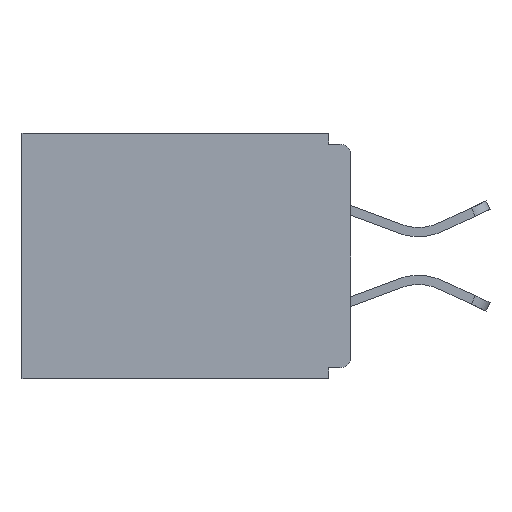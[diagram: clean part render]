
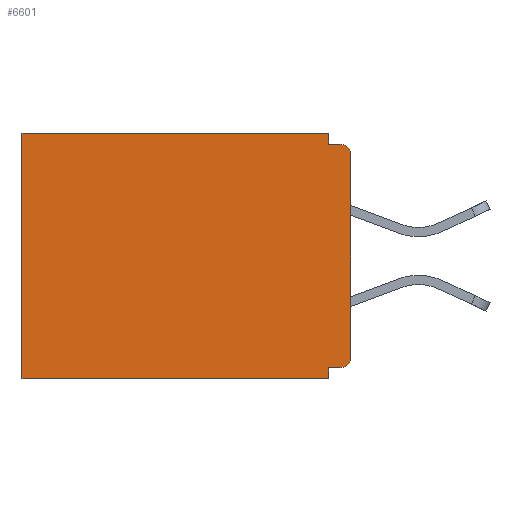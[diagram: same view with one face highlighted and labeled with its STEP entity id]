
A CAD part, left-side view. The second image highlights one B-rep face of the part: STEP entity #6601.
In plain terms, the highlighted planar face has unit normal (-1, 0, 0).
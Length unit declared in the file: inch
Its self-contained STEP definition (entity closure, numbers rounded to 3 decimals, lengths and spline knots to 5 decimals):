
#123 = ORIENTED_EDGE ( 'NONE', *, *, #4149, .T. ) ;
#448 = LINE ( 'NONE', #15597, #10833 ) ;
#1018 = VERTEX_POINT ( 'NONE', #11713 ) ;
#1474 = EDGE_CURVE ( 'NONE', #13057, #2625, #13930, .T. ) ;
#1483 = EDGE_CURVE ( 'NONE', #7050, #9009, #9162, .T. ) ;
#1697 = VECTOR ( 'NONE', #12200, 39.37008 ) ;
#1750 = ORIENTED_EDGE ( 'NONE', *, *, #1483, .F. ) ;
#1841 = CARTESIAN_POINT ( 'NONE',  ( 0.298, 0., 0. ) ) ;
#1875 = VERTEX_POINT ( 'NONE', #3403 ) ;
#2086 = VERTEX_POINT ( 'NONE', #8594 ) ;
#2167 = ORIENTED_EDGE ( 'NONE', *, *, #2631, .F. ) ;
#2180 = CARTESIAN_POINT ( 'NONE',  ( 0.298, 0.46, -0.343 ) ) ;
#2319 = EDGE_CURVE ( 'NONE', #2086, #2996, #7268, .T. ) ;
#2546 = CARTESIAN_POINT ( 'NONE',  ( 0.298, 0., -0.015 ) ) ;
#2625 = VERTEX_POINT ( 'NONE', #5734 ) ;
#2631 = EDGE_CURVE ( 'NONE', #13057, #6788, #15055, .T. ) ;
#2850 = LINE ( 'NONE', #2546, #1697 ) ;
#2859 = EDGE_CURVE ( 'NONE', #1018, #2996, #11800, .T. ) ;
#2996 = VERTEX_POINT ( 'NONE', #11262 ) ;
#3275 = EDGE_CURVE ( 'NONE', #2086, #15191, #10846, .T. ) ;
#3403 = CARTESIAN_POINT ( 'NONE',  ( 0.298, 0.015, -0.015 ) ) ;
#3463 = DIRECTION ( 'NONE',  ( 0., 1., 0. ) ) ;
#3483 = DIRECTION ( 'NONE',  ( 0., 0., -1. ) ) ;
#3580 = CARTESIAN_POINT ( 'NONE',  ( 0.298, 0.015, -0.313 ) ) ;
#4040 = LINE ( 'NONE', #11804, #10444 ) ;
#4149 = EDGE_CURVE ( 'NONE', #1018, #1875, #11959, .T. ) ;
#4512 = DIRECTION ( 'NONE',  ( -1., 0., 0. ) ) ;
#4696 = CARTESIAN_POINT ( 'NONE',  ( 0.298, 0., 0. ) ) ;
#4710 = DIRECTION ( 'NONE',  ( 0., 0., -1. ) ) ;
#5500 = CARTESIAN_POINT ( 'NONE',  ( 0.298, 0.031, -0.015 ) ) ;
#5665 = ORIENTED_EDGE ( 'NONE', *, *, #2319, .T. ) ;
#5734 = CARTESIAN_POINT ( 'NONE',  ( 0.298, 0.46, 0. ) ) ;
#5794 = DIRECTION ( 'NONE',  ( 0., 1., 0. ) ) ;
#5813 = DIRECTION ( 'NONE',  ( -1., 0., 0. ) ) ;
#6601 = ADVANCED_FACE ( 'NONE', ( #8647 ), #6876, .F. ) ;
#6788 = VERTEX_POINT ( 'NONE', #5500 ) ;
#6876 = PLANE ( 'NONE',  #10411 ) ;
#7050 = VERTEX_POINT ( 'NONE', #12848 ) ;
#7137 = EDGE_LOOP ( 'NONE', ( #123, #11182, #2167, #12287, #9486, #1750, #15047, #9133, #5665, #9840 ) ) ;
#7268 = CIRCLE ( 'NONE', #7648, 0.015 ) ;
#7577 = CARTESIAN_POINT ( 'NONE',  ( 0.298, 0.031, 0. ) ) ;
#7648 = AXIS2_PLACEMENT_3D ( 'NONE', #3580, #5813, #4710 ) ;
#7831 = VECTOR ( 'NONE', #8062, 39.37008 ) ;
#7996 = VECTOR ( 'NONE', #8225, 39.37008 ) ;
#8009 = CARTESIAN_POINT ( 'NONE',  ( 0.298, 0.031, -0.343 ) ) ;
#8062 = DIRECTION ( 'NONE',  ( 0., 0., -1. ) ) ;
#8225 = DIRECTION ( 'NONE',  ( 0., 1., 0. ) ) ;
#8379 = CARTESIAN_POINT ( 'NONE',  ( 0.298, 0., -0.328 ) ) ;
#8381 = VECTOR ( 'NONE', #9684, 39.37008 ) ;
#8594 = CARTESIAN_POINT ( 'NONE',  ( 0.298, 0.015, -0.328 ) ) ;
#8647 = FACE_OUTER_BOUND ( 'NONE', #7137, .T. ) ;
#8824 = EDGE_CURVE ( 'NONE', #2625, #9009, #448, .T. ) ;
#9009 = VERTEX_POINT ( 'NONE', #2180 ) ;
#9051 = AXIS2_PLACEMENT_3D ( 'NONE', #15288, #4512, #10525 ) ;
#9133 = ORIENTED_EDGE ( 'NONE', *, *, #3275, .F. ) ;
#9162 = LINE ( 'NONE', #10620, #9722 ) ;
#9486 = ORIENTED_EDGE ( 'NONE', *, *, #8824, .T. ) ;
#9684 = DIRECTION ( 'NONE',  ( 0., 0., -1. ) ) ;
#9722 = VECTOR ( 'NONE', #3463, 39.37008 ) ;
#9840 = ORIENTED_EDGE ( 'NONE', *, *, #2859, .F. ) ;
#10276 = DIRECTION ( 'NONE',  ( 1., 0., 0. ) ) ;
#10411 = AXIS2_PLACEMENT_3D ( 'NONE', #1841, #10276, #11617 ) ;
#10444 = VECTOR ( 'NONE', #3483, 39.37008 ) ;
#10525 = DIRECTION ( 'NONE',  ( 0., 0., -1. ) ) ;
#10620 = CARTESIAN_POINT ( 'NONE',  ( 0.298, 0., -0.343 ) ) ;
#10833 = VECTOR ( 'NONE', #12140, 39.37008 ) ;
#10846 = LINE ( 'NONE', #8379, #7996 ) ;
#11182 = ORIENTED_EDGE ( 'NONE', *, *, #11357, .F. ) ;
#11262 = CARTESIAN_POINT ( 'NONE',  ( 0.298, 0., -0.313 ) ) ;
#11357 = EDGE_CURVE ( 'NONE', #6788, #1875, #2850, .T. ) ;
#11617 = DIRECTION ( 'NONE',  ( 0., 0., -1. ) ) ;
#11713 = CARTESIAN_POINT ( 'NONE',  ( 0.298, 0., -0.03 ) ) ;
#11800 = LINE ( 'NONE', #11935, #8381 ) ;
#11804 = CARTESIAN_POINT ( 'NONE',  ( 0.298, 0.031, -0.343 ) ) ;
#11935 = CARTESIAN_POINT ( 'NONE',  ( 0.298, 0., 0. ) ) ;
#11959 = CIRCLE ( 'NONE', #9051, 0.015 ) ;
#12015 = VECTOR ( 'NONE', #5794, 39.37008 ) ;
#12140 = DIRECTION ( 'NONE',  ( 0., 0., -1. ) ) ;
#12200 = DIRECTION ( 'NONE',  ( 0., -1., 0. ) ) ;
#12287 = ORIENTED_EDGE ( 'NONE', *, *, #1474, .T. ) ;
#12848 = CARTESIAN_POINT ( 'NONE',  ( 0.298, 0.031, -0.343 ) ) ;
#13057 = VERTEX_POINT ( 'NONE', #7577 ) ;
#13930 = LINE ( 'NONE', #4696, #12015 ) ;
#14618 = CARTESIAN_POINT ( 'NONE',  ( 0.298, 0.031, -0.328 ) ) ;
#15038 = EDGE_CURVE ( 'NONE', #15191, #7050, #4040, .T. ) ;
#15047 = ORIENTED_EDGE ( 'NONE', *, *, #15038, .F. ) ;
#15055 = LINE ( 'NONE', #8009, #7831 ) ;
#15191 = VERTEX_POINT ( 'NONE', #14618 ) ;
#15288 = CARTESIAN_POINT ( 'NONE',  ( 0.298, 0.015, -0.03 ) ) ;
#15597 = CARTESIAN_POINT ( 'NONE',  ( 0.298, 0.46, 0. ) ) ;
